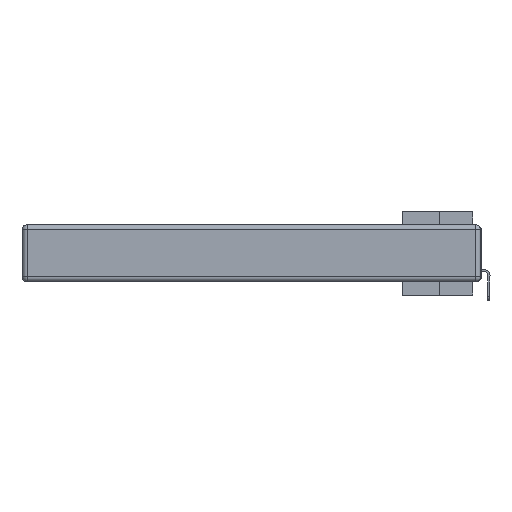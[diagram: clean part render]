
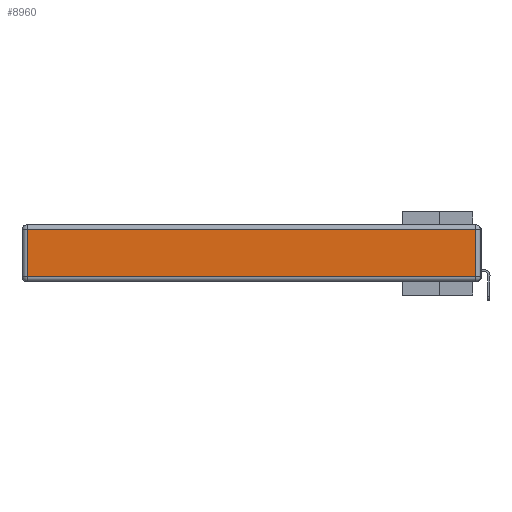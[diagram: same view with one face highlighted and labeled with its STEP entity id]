
A CAD part, left-side view. The second image highlights one B-rep face of the part: STEP entity #8960.
In plain terms, the highlighted planar face has unit normal (-1, 0, 0).
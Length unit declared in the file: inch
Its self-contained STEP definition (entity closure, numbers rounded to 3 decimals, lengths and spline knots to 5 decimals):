
#618 = DIRECTION ( 'NONE',  ( 0., 1., 0. ) ) ;
#733 = LINE ( 'NONE', #23018, #25522 ) ;
#1659 = VECTOR ( 'NONE', #30769, 39.37008 ) ;
#3300 = CARTESIAN_POINT ( 'NONE',  ( 0., 2.72, -0.313 ) ) ;
#3450 = EDGE_CURVE ( 'NONE', #6048, #21821, #8137, .T. ) ;
#4343 = VECTOR ( 'NONE', #19152, 39.37008 ) ;
#4999 = EDGE_CURVE ( 'NONE', #20269, #6048, #733, .T. ) ;
#6048 = VERTEX_POINT ( 'NONE', #6759 ) ;
#6394 = EDGE_CURVE ( 'NONE', #21821, #16470, #16340, .T. ) ;
#6648 = CARTESIAN_POINT ( 'NONE',  ( 0., 0.03, -0.343 ) ) ;
#6759 = CARTESIAN_POINT ( 'NONE',  ( 0., 0.03, -0.313 ) ) ;
#6832 = FACE_OUTER_BOUND ( 'NONE', #17373, .T. ) ;
#8137 = LINE ( 'NONE', #6648, #1659 ) ;
#8960 = ADVANCED_FACE ( 'NONE', ( #6832 ), #11069, .T. ) ;
#9276 = LINE ( 'NONE', #28675, #4343 ) ;
#9867 = ORIENTED_EDGE ( 'NONE', *, *, #4999, .T. ) ;
#11069 = PLANE ( 'NONE',  #28632 ) ;
#12762 = CARTESIAN_POINT ( 'NONE',  ( 0., 2.75, -0.03 ) ) ;
#14066 = ORIENTED_EDGE ( 'NONE', *, *, #17840, .T. ) ;
#16340 = LINE ( 'NONE', #12762, #17828 ) ;
#16470 = VERTEX_POINT ( 'NONE', #29541 ) ;
#17373 = EDGE_LOOP ( 'NONE', ( #9867, #28476, #27360, #14066 ) ) ;
#17828 = VECTOR ( 'NONE', #618, 39.37008 ) ;
#17840 = EDGE_CURVE ( 'NONE', #16470, #20269, #9276, .T. ) ;
#18349 = CARTESIAN_POINT ( 'NONE',  ( 0., 0., -0.343 ) ) ;
#18652 = DIRECTION ( 'NONE',  ( 0., -1., 0. ) ) ;
#19152 = DIRECTION ( 'NONE',  ( 0., 0., -1. ) ) ;
#20269 = VERTEX_POINT ( 'NONE', #3300 ) ;
#20844 = CARTESIAN_POINT ( 'NONE',  ( 0., 0.03, -0.03 ) ) ;
#21821 = VERTEX_POINT ( 'NONE', #20844 ) ;
#23018 = CARTESIAN_POINT ( 'NONE',  ( 0., 0., -0.313 ) ) ;
#25522 = VECTOR ( 'NONE', #18652, 39.37008 ) ;
#27360 = ORIENTED_EDGE ( 'NONE', *, *, #6394, .T. ) ;
#28067 = DIRECTION ( 'NONE',  ( -1., 0., 0. ) ) ;
#28476 = ORIENTED_EDGE ( 'NONE', *, *, #3450, .T. ) ;
#28632 = AXIS2_PLACEMENT_3D ( 'NONE', #18349, #28067, #30478 ) ;
#28675 = CARTESIAN_POINT ( 'NONE',  ( 0., 2.72, -0.343 ) ) ;
#29541 = CARTESIAN_POINT ( 'NONE',  ( 0., 2.72, -0.03 ) ) ;
#30478 = DIRECTION ( 'NONE',  ( 0., 0., 1. ) ) ;
#30769 = DIRECTION ( 'NONE',  ( 0., 0., 1. ) ) ;
